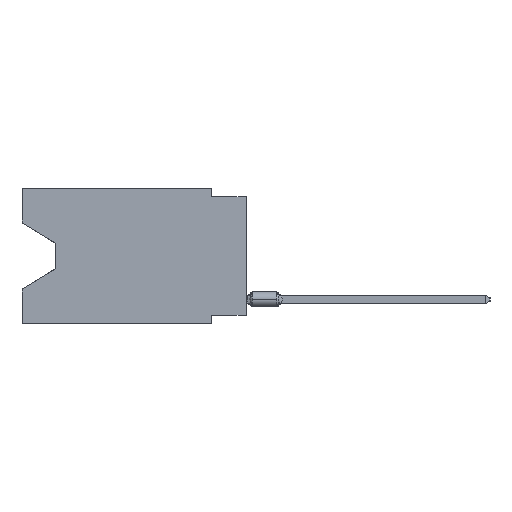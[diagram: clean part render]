
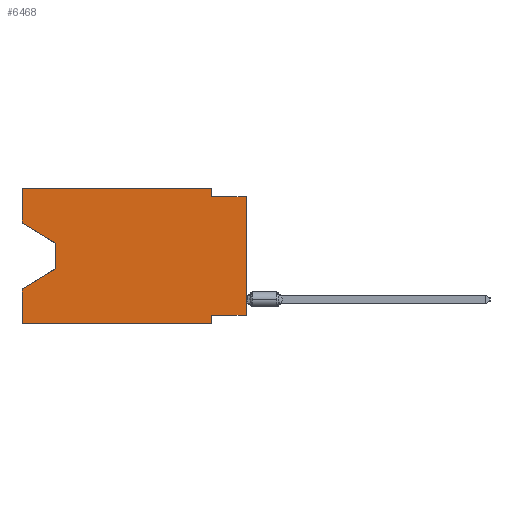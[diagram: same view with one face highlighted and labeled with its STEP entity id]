
A CAD part, left-side view. The second image highlights one B-rep face of the part: STEP entity #6468.
In plain terms, the highlighted planar face has unit normal (-1, 0, 0).
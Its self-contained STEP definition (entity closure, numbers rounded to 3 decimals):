
#495 = VERTEX_POINT ( 'NONE', #34337 ) ;
#1311 = VERTEX_POINT ( 'NONE', #38603 ) ;
#1644 = VECTOR ( 'NONE', #40093, 1000. ) ;
#1922 = EDGE_CURVE ( 'NONE', #46186, #19765, #7210, .T. ) ;
#2024 = CARTESIAN_POINT ( 'NONE',  ( 0., 16.383, -2.546 ) ) ;
#2220 = FACE_OUTER_BOUND ( 'NONE', #21468, .T. ) ;
#2582 = CARTESIAN_POINT ( 'NONE',  ( 0., 0., -0.635 ) ) ;
#2991 = LINE ( 'NONE', #43753, #41286 ) ;
#3262 = EDGE_CURVE ( 'NONE', #1311, #495, #37516, .T. ) ;
#3677 = VECTOR ( 'NONE', #28933, 1000. ) ;
#3813 = CARTESIAN_POINT ( 'NONE',  ( 0., 16.383, 0. ) ) ;
#4426 = VERTEX_POINT ( 'NONE', #2582 ) ;
#6005 = VERTEX_POINT ( 'NONE', #29044 ) ;
#6468 = ADVANCED_FACE ( 'NONE', ( #2220 ), #52053, .F. ) ;
#6524 = VECTOR ( 'NONE', #39423, 1000. ) ;
#6538 = DIRECTION ( 'NONE',  ( 0., 0., 1. ) ) ;
#6758 = LINE ( 'NONE', #38164, #32932 ) ;
#7210 = LINE ( 'NONE', #25099, #3677 ) ;
#7983 = LINE ( 'NONE', #51409, #30988 ) ;
#8761 = VERTEX_POINT ( 'NONE', #40025 ) ;
#9099 = EDGE_CURVE ( 'NONE', #1311, #6005, #10953, .T. ) ;
#9826 = CARTESIAN_POINT ( 'NONE',  ( 0., 16.383, -9.906 ) ) ;
#10534 = DIRECTION ( 'NONE',  ( 0., -0.855, -0.519 ) ) ;
#10715 = CARTESIAN_POINT ( 'NONE',  ( 0., 2.54, -9.271 ) ) ;
#10784 = ORIENTED_EDGE ( 'NONE', *, *, #46089, .T. ) ;
#10953 = LINE ( 'NONE', #28850, #41783 ) ;
#11520 = LINE ( 'NONE', #47283, #11716 ) ;
#11716 = VECTOR ( 'NONE', #51124, 1000. ) ;
#13482 = LINE ( 'NONE', #3813, #45903 ) ;
#13674 = CARTESIAN_POINT ( 'NONE',  ( 0., 16.383, -7.36 ) ) ;
#13902 = ORIENTED_EDGE ( 'NONE', *, *, #1922, .F. ) ;
#14447 = DIRECTION ( 'NONE',  ( 0., 0., 1. ) ) ;
#14558 = EDGE_CURVE ( 'NONE', #17349, #53198, #11520, .T. ) ;
#15034 = CARTESIAN_POINT ( 'NONE',  ( 0., 0., 0. ) ) ;
#16892 = DIRECTION ( 'NONE',  ( 0., 0., -1. ) ) ;
#17349 = VERTEX_POINT ( 'NONE', #9826 ) ;
#19444 = EDGE_CURVE ( 'NONE', #495, #56290, #33659, .T. ) ;
#19765 = VERTEX_POINT ( 'NONE', #10715 ) ;
#20035 = DIRECTION ( 'NONE',  ( 0., 0., -1. ) ) ;
#20112 = CARTESIAN_POINT ( 'NONE',  ( 0., 2.54, 0. ) ) ;
#20267 = EDGE_CURVE ( 'NONE', #46186, #4426, #32056, .T. ) ;
#20966 = CARTESIAN_POINT ( 'NONE',  ( 0., 16.383, 0. ) ) ;
#21468 = EDGE_LOOP ( 'NONE', ( #38674, #30940, #10784, #45754, #34283, #36928, #13902, #42481, #42870, #30464, #26943, #24198 ) ) ;
#21814 = LINE ( 'NONE', #30610, #6524 ) ;
#24198 = ORIENTED_EDGE ( 'NONE', *, *, #9099, .F. ) ;
#25099 = CARTESIAN_POINT ( 'NONE',  ( 0., 0., -9.271 ) ) ;
#25369 = EDGE_CURVE ( 'NONE', #17349, #57557, #21814, .T. ) ;
#26873 = EDGE_CURVE ( 'NONE', #8761, #4426, #2991, .T. ) ;
#26943 = ORIENTED_EDGE ( 'NONE', *, *, #55574, .F. ) ;
#26972 = DIRECTION ( 'NONE',  ( 0., -1., 0. ) ) ;
#28850 = CARTESIAN_POINT ( 'NONE',  ( 0., 16.383, 0. ) ) ;
#28933 = DIRECTION ( 'NONE',  ( 0., 1., 0. ) ) ;
#29044 = CARTESIAN_POINT ( 'NONE',  ( 0., 16.383, 0. ) ) ;
#29723 = CARTESIAN_POINT ( 'NONE',  ( 0., 13.97, -5.893 ) ) ;
#30464 = ORIENTED_EDGE ( 'NONE', *, *, #45783, .F. ) ;
#30610 = CARTESIAN_POINT ( 'NONE',  ( 0., 16.383, -9.906 ) ) ;
#30940 = ORIENTED_EDGE ( 'NONE', *, *, #19444, .T. ) ;
#30988 = VECTOR ( 'NONE', #20035, 1000. ) ;
#32056 = LINE ( 'NONE', #15034, #43993 ) ;
#32932 = VECTOR ( 'NONE', #33465, 1000. ) ;
#33465 = DIRECTION ( 'NONE',  ( 0., 0.855, -0.519 ) ) ;
#33659 = LINE ( 'NONE', #38631, #38318 ) ;
#34283 = ORIENTED_EDGE ( 'NONE', *, *, #25369, .T. ) ;
#34337 = CARTESIAN_POINT ( 'NONE',  ( 0., 13.97, -4.013 ) ) ;
#36928 = ORIENTED_EDGE ( 'NONE', *, *, #53134, .F. ) ;
#37472 = CARTESIAN_POINT ( 'NONE',  ( 0., 2.54, -9.906 ) ) ;
#37516 = LINE ( 'NONE', #2024, #37527 ) ;
#37527 = VECTOR ( 'NONE', #10534, 1000. ) ;
#38013 = DIRECTION ( 'NONE',  ( 0., 0., -1. ) ) ;
#38164 = CARTESIAN_POINT ( 'NONE',  ( 0., 13.97, -5.893 ) ) ;
#38318 = VECTOR ( 'NONE', #16892, 1000. ) ;
#38603 = CARTESIAN_POINT ( 'NONE',  ( 0., 16.383, -2.546 ) ) ;
#38631 = CARTESIAN_POINT ( 'NONE',  ( 0., 13.97, -4.013 ) ) ;
#38674 = ORIENTED_EDGE ( 'NONE', *, *, #3262, .T. ) ;
#39423 = DIRECTION ( 'NONE',  ( 0., -1., 0. ) ) ;
#40025 = CARTESIAN_POINT ( 'NONE',  ( 0., 2.54, -0.635 ) ) ;
#40093 = DIRECTION ( 'NONE',  ( 0., 0., -1. ) ) ;
#41286 = VECTOR ( 'NONE', #52250, 1000. ) ;
#41783 = VECTOR ( 'NONE', #6538, 1000. ) ;
#42481 = ORIENTED_EDGE ( 'NONE', *, *, #20267, .T. ) ;
#42590 = AXIS2_PLACEMENT_3D ( 'NONE', #20966, #55600, #38013 ) ;
#42870 = ORIENTED_EDGE ( 'NONE', *, *, #26873, .F. ) ;
#43753 = CARTESIAN_POINT ( 'NONE',  ( 0., 0., -0.635 ) ) ;
#43993 = VECTOR ( 'NONE', #14447, 1000. ) ;
#45754 = ORIENTED_EDGE ( 'NONE', *, *, #14558, .F. ) ;
#45783 = EDGE_CURVE ( 'NONE', #53273, #8761, #7983, .T. ) ;
#45903 = VECTOR ( 'NONE', #26972, 1000. ) ;
#46089 = EDGE_CURVE ( 'NONE', #56290, #53198, #6758, .T. ) ;
#46186 = VERTEX_POINT ( 'NONE', #55751 ) ;
#47283 = CARTESIAN_POINT ( 'NONE',  ( 0., 16.383, 0. ) ) ;
#50037 = CARTESIAN_POINT ( 'NONE',  ( 0., 2.54, -9.906 ) ) ;
#51124 = DIRECTION ( 'NONE',  ( 0., 0., 1. ) ) ;
#51409 = CARTESIAN_POINT ( 'NONE',  ( 0., 2.54, 0. ) ) ;
#52053 = PLANE ( 'NONE',  #42590 ) ;
#52250 = DIRECTION ( 'NONE',  ( 0., -1., 0. ) ) ;
#53134 = EDGE_CURVE ( 'NONE', #19765, #57557, #53260, .T. ) ;
#53198 = VERTEX_POINT ( 'NONE', #13674 ) ;
#53260 = LINE ( 'NONE', #50037, #1644 ) ;
#53273 = VERTEX_POINT ( 'NONE', #20112 ) ;
#55574 = EDGE_CURVE ( 'NONE', #6005, #53273, #13482, .T. ) ;
#55600 = DIRECTION ( 'NONE',  ( 1., 0., 0. ) ) ;
#55751 = CARTESIAN_POINT ( 'NONE',  ( 0., 0., -9.271 ) ) ;
#56290 = VERTEX_POINT ( 'NONE', #29723 ) ;
#57557 = VERTEX_POINT ( 'NONE', #37472 ) ;
